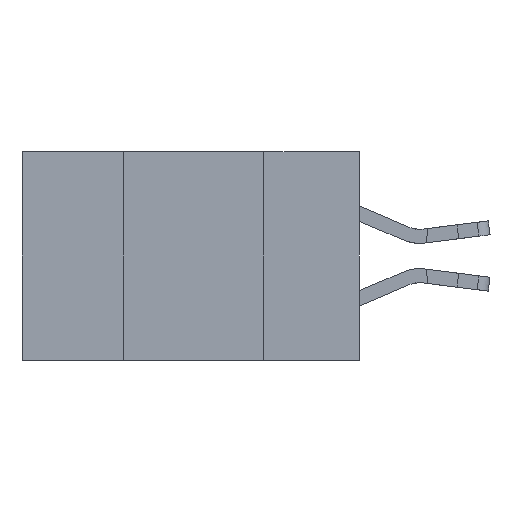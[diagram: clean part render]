
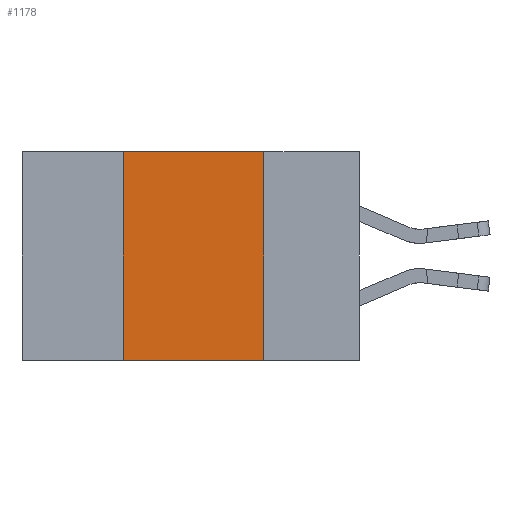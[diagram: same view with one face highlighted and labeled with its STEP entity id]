
A CAD part, left-side view. The second image highlights one B-rep face of the part: STEP entity #1178.
In plain terms, the highlighted planar face has unit normal (-1, 0, 0).
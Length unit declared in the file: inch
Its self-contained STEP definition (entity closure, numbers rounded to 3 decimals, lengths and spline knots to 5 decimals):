
#844 = LINE ( 'NONE', #3023, #6973 ) ;
#1178 = ADVANCED_FACE ( 'NONE', ( #7656 ), #4356, .F. ) ;
#1260 = AXIS2_PLACEMENT_3D ( 'NONE', #8375, #27994, #10762 ) ;
#3023 = CARTESIAN_POINT ( 'NONE',  ( 0., 0.6, 0. ) ) ;
#4356 = PLANE ( 'NONE',  #1260 ) ;
#6973 = VECTOR ( 'NONE', #16255, 39.37008 ) ;
#7018 = CARTESIAN_POINT ( 'NONE',  ( 0., 0.17, -0.37 ) ) ;
#7230 = VECTOR ( 'NONE', #14960, 39.37008 ) ;
#7656 = FACE_OUTER_BOUND ( 'NONE', #23331, .T. ) ;
#8046 = CARTESIAN_POINT ( 'NONE',  ( 0., 0.42, 0. ) ) ;
#8375 = CARTESIAN_POINT ( 'NONE',  ( 0., 0.6, 0. ) ) ;
#9008 = VERTEX_POINT ( 'NONE', #7018 ) ;
#10258 = VECTOR ( 'NONE', #16739, 39.37008 ) ;
#10762 = DIRECTION ( 'NONE',  ( 0., 0., -1. ) ) ;
#10875 = CARTESIAN_POINT ( 'NONE',  ( 0., 0.42, -0.37 ) ) ;
#11258 = LINE ( 'NONE', #21216, #10258 ) ;
#11912 = VERTEX_POINT ( 'NONE', #8046 ) ;
#12011 = ORIENTED_EDGE ( 'NONE', *, *, #20717, .F. ) ;
#13091 = LINE ( 'NONE', #23373, #7230 ) ;
#13636 = DIRECTION ( 'NONE',  ( 0., 0., -1. ) ) ;
#14960 = DIRECTION ( 'NONE',  ( 0., -1., 0. ) ) ;
#15020 = VECTOR ( 'NONE', #13636, 39.37008 ) ;
#15171 = CARTESIAN_POINT ( 'NONE',  ( 0., 0.17, 0. ) ) ;
#15640 = CARTESIAN_POINT ( 'NONE',  ( 0., 0.17, 0. ) ) ;
#15912 = VERTEX_POINT ( 'NONE', #10875 ) ;
#16255 = DIRECTION ( 'NONE',  ( 0., -1., 0. ) ) ;
#16739 = DIRECTION ( 'NONE',  ( 0., 0., 1. ) ) ;
#16935 = EDGE_CURVE ( 'NONE', #15912, #9008, #13091, .T. ) ;
#19581 = VERTEX_POINT ( 'NONE', #15640 ) ;
#19901 = EDGE_CURVE ( 'NONE', #15912, #11912, #11258, .T. ) ;
#20343 = ORIENTED_EDGE ( 'NONE', *, *, #16935, .T. ) ;
#20717 = EDGE_CURVE ( 'NONE', #19581, #9008, #26551, .T. ) ;
#21216 = CARTESIAN_POINT ( 'NONE',  ( 0., 0.42, 0. ) ) ;
#21572 = ORIENTED_EDGE ( 'NONE', *, *, #23565, .F. ) ;
#23331 = EDGE_LOOP ( 'NONE', ( #12011, #21572, #23555, #20343 ) ) ;
#23373 = CARTESIAN_POINT ( 'NONE',  ( 0., 0.6, -0.37 ) ) ;
#23555 = ORIENTED_EDGE ( 'NONE', *, *, #19901, .F. ) ;
#23565 = EDGE_CURVE ( 'NONE', #11912, #19581, #844, .T. ) ;
#26551 = LINE ( 'NONE', #15171, #15020 ) ;
#27994 = DIRECTION ( 'NONE',  ( 1., 0., 0. ) ) ;
